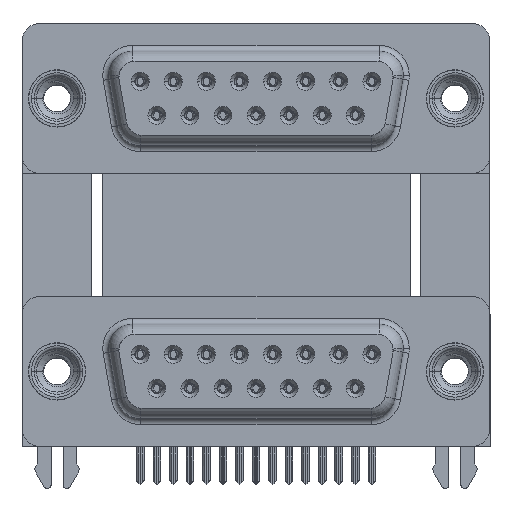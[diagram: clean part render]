
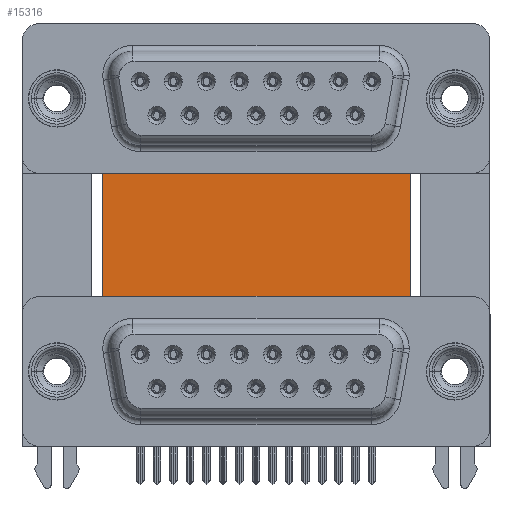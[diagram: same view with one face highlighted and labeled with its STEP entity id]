
A CAD part, top view. The second image highlights one B-rep face of the part: STEP entity #15316.
In plain terms, the highlighted planar face has unit normal (0, 0, 1).
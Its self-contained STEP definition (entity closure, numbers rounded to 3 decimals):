
#3974 = CARTESIAN_POINT ( 'NONE',  ( 29.58, 16.585, -12. ) ) ;
#5321 = EDGE_CURVE ( 'NONE', #8580, #13993, #36577, .T. ) ;
#5977 = ORIENTED_EDGE ( 'NONE', *, *, #46523, .T. ) ;
#6014 = EDGE_CURVE ( 'NONE', #12311, #50270, #33265, .T. ) ;
#8580 = VERTEX_POINT ( 'NONE', #43275 ) ;
#9171 = DIRECTION ( 'NONE',  ( 1., 0., 0. ) ) ;
#9427 = CARTESIAN_POINT ( 'NONE',  ( 3.79, -3.735, -12. ) ) ;
#9538 = AXIS2_PLACEMENT_3D ( 'NONE', #21891, #45479, #37522 ) ;
#9743 = ORIENTED_EDGE ( 'NONE', *, *, #21210, .F. ) ;
#12311 = VERTEX_POINT ( 'NONE', #31452 ) ;
#13792 = VECTOR ( 'NONE', #39834, 1000. ) ;
#13809 = DIRECTION ( 'NONE',  ( 1., 0., 0. ) ) ;
#13993 = VERTEX_POINT ( 'NONE', #40367 ) ;
#14476 = FACE_OUTER_BOUND ( 'NONE', #26259, .T. ) ;
#15316 = ADVANCED_FACE ( 'NONE', ( #14476 ), #36332, .F. ) ;
#15325 = LINE ( 'NONE', #30937, #49409 ) ;
#18289 = ORIENTED_EDGE ( 'NONE', *, *, #5321, .T. ) ;
#21210 = EDGE_CURVE ( 'NONE', #50270, #13993, #24190, .T. ) ;
#21891 = CARTESIAN_POINT ( 'NONE',  ( 3.79, 16.585, -12. ) ) ;
#24190 = LINE ( 'NONE', #3974, #13792 ) ;
#26259 = EDGE_LOOP ( 'NONE', ( #18289, #9743, #33997, #5977 ) ) ;
#27080 = DIRECTION ( 'NONE',  ( 0., -1., 0. ) ) ;
#29231 = CARTESIAN_POINT ( 'NONE',  ( 29.58, 16.585, -12. ) ) ;
#29811 = VECTOR ( 'NONE', #13809, 1000. ) ;
#30937 = CARTESIAN_POINT ( 'NONE',  ( 3.79, 16.585, -12. ) ) ;
#31452 = CARTESIAN_POINT ( 'NONE',  ( 3.79, 16.585, -12. ) ) ;
#33265 = LINE ( 'NONE', #45321, #29811 ) ;
#33997 = ORIENTED_EDGE ( 'NONE', *, *, #6014, .F. ) ;
#36332 = PLANE ( 'NONE',  #9538 ) ;
#36577 = LINE ( 'NONE', #9427, #47391 ) ;
#37522 = DIRECTION ( 'NONE',  ( -1., 0., 0. ) ) ;
#39834 = DIRECTION ( 'NONE',  ( 0., -1., 0. ) ) ;
#40367 = CARTESIAN_POINT ( 'NONE',  ( 29.58, -3.735, -12. ) ) ;
#43275 = CARTESIAN_POINT ( 'NONE',  ( 3.79, -3.735, -12. ) ) ;
#45321 = CARTESIAN_POINT ( 'NONE',  ( 3.79, 16.585, -12. ) ) ;
#45479 = DIRECTION ( 'NONE',  ( 0., 0., -1. ) ) ;
#46523 = EDGE_CURVE ( 'NONE', #12311, #8580, #15325, .T. ) ;
#47391 = VECTOR ( 'NONE', #9171, 1000. ) ;
#49409 = VECTOR ( 'NONE', #27080, 1000. ) ;
#50270 = VERTEX_POINT ( 'NONE', #29231 ) ;
